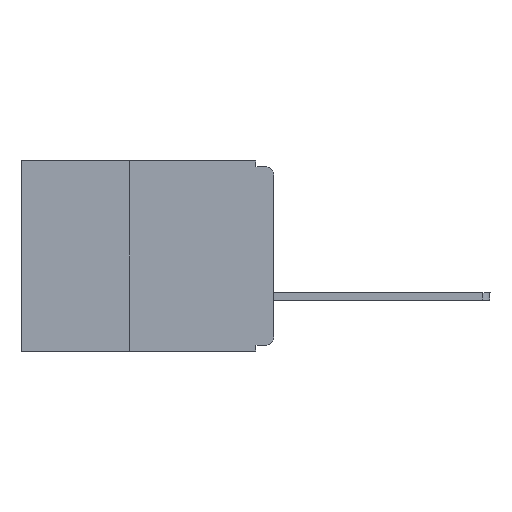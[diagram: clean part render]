
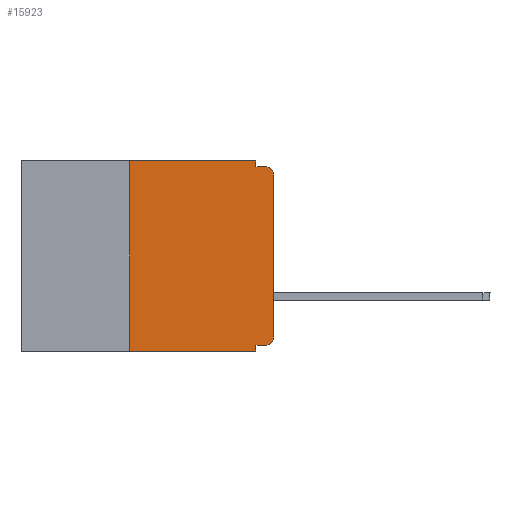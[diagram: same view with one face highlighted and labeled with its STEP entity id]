
A CAD part, left-side view. The second image highlights one B-rep face of the part: STEP entity #15923.
In plain terms, the highlighted planar face has unit normal (-1, 0, 0).
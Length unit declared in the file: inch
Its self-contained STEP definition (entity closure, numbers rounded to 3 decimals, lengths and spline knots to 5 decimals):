
#31 = VECTOR ( 'NONE', #1670, 39.37008 ) ;
#232 = CARTESIAN_POINT ( 'NONE',  ( 0., 0., -0.305 ) ) ;
#716 = CARTESIAN_POINT ( 'NONE',  ( 0., 0.031, -0.01 ) ) ;
#1041 = DIRECTION ( 'NONE',  ( -1., 0., 0. ) ) ;
#1102 = DIRECTION ( 'NONE',  ( 0., 0., -1. ) ) ;
#1212 = ORIENTED_EDGE ( 'NONE', *, *, #5868, .F. ) ;
#1413 = EDGE_CURVE ( 'NONE', #12002, #6217, #3180, .T. ) ;
#1670 = DIRECTION ( 'NONE',  ( 0., 0., 1. ) ) ;
#2000 = LINE ( 'NONE', #8770, #11745 ) ;
#2105 = EDGE_LOOP ( 'NONE', ( #5116, #5267, #5777, #15504, #9404, #3932, #16204, #1212, #5912, #4914 ) ) ;
#2381 = DIRECTION ( 'NONE',  ( 0., 0., -1. ) ) ;
#2387 = DIRECTION ( 'NONE',  ( 1., 0., 0. ) ) ;
#2627 = VERTEX_POINT ( 'NONE', #6374 ) ;
#2690 = CARTESIAN_POINT ( 'NONE',  ( 0., 0.015, -0.305 ) ) ;
#2705 = EDGE_CURVE ( 'NONE', #2627, #14074, #12672, .T. ) ;
#2966 = EDGE_CURVE ( 'NONE', #9240, #2627, #12854, .T. ) ;
#3180 = LINE ( 'NONE', #13560, #15653 ) ;
#3362 = VECTOR ( 'NONE', #7516, 39.37008 ) ;
#3506 = CARTESIAN_POINT ( 'NONE',  ( 0., 0.015, -0.01 ) ) ;
#3932 = ORIENTED_EDGE ( 'NONE', *, *, #13009, .F. ) ;
#4101 = EDGE_CURVE ( 'NONE', #11292, #12118, #8867, .T. ) ;
#4219 = LINE ( 'NONE', #9597, #31 ) ;
#4336 = FACE_OUTER_BOUND ( 'NONE', #2105, .T. ) ;
#4453 = DIRECTION ( 'NONE',  ( 0., 0., 1. ) ) ;
#4914 = ORIENTED_EDGE ( 'NONE', *, *, #14160, .T. ) ;
#5116 = ORIENTED_EDGE ( 'NONE', *, *, #2966, .T. ) ;
#5264 = EDGE_CURVE ( 'NONE', #12173, #6112, #2000, .T. ) ;
#5267 = ORIENTED_EDGE ( 'NONE', *, *, #2705, .T. ) ;
#5777 = ORIENTED_EDGE ( 'NONE', *, *, #9657, .F. ) ;
#5868 = EDGE_CURVE ( 'NONE', #6217, #6112, #9236, .T. ) ;
#5912 = ORIENTED_EDGE ( 'NONE', *, *, #1413, .F. ) ;
#6054 = CARTESIAN_POINT ( 'NONE',  ( 0., 0.031, -0.32 ) ) ;
#6080 = DIRECTION ( 'NONE',  ( 0., -1., 0. ) ) ;
#6112 = VERTEX_POINT ( 'NONE', #16605 ) ;
#6217 = VERTEX_POINT ( 'NONE', #6054 ) ;
#6374 = CARTESIAN_POINT ( 'NONE',  ( 0., 0., -0.025 ) ) ;
#6806 = DIRECTION ( 'NONE',  ( 0., 0., -1. ) ) ;
#7268 = DIRECTION ( 'NONE',  ( 0., -1., 0. ) ) ;
#7516 = DIRECTION ( 'NONE',  ( 0., -1., 0. ) ) ;
#7982 = VERTEX_POINT ( 'NONE', #716 ) ;
#8004 = DIRECTION ( 'NONE',  ( -1., 0., 0. ) ) ;
#8770 = CARTESIAN_POINT ( 'NONE',  ( 0., 0.437, -0.33 ) ) ;
#8867 = LINE ( 'NONE', #14034, #9700 ) ;
#8929 = CARTESIAN_POINT ( 'NONE',  ( 0., 0.015, -0.025 ) ) ;
#9201 = CARTESIAN_POINT ( 'NONE',  ( 0., 0.031, 0. ) ) ;
#9236 = LINE ( 'NONE', #11000, #12559 ) ;
#9240 = VERTEX_POINT ( 'NONE', #232 ) ;
#9404 = ORIENTED_EDGE ( 'NONE', *, *, #4101, .F. ) ;
#9597 = CARTESIAN_POINT ( 'NONE',  ( 0., 0.25, -0.33 ) ) ;
#9657 = EDGE_CURVE ( 'NONE', #7982, #14074, #15204, .T. ) ;
#9700 = VECTOR ( 'NONE', #6080, 39.37008 ) ;
#9705 = CARTESIAN_POINT ( 'NONE',  ( 0., 0.25, 0. ) ) ;
#10078 = CARTESIAN_POINT ( 'NONE',  ( 0., 0.25, -0.33 ) ) ;
#10204 = CARTESIAN_POINT ( 'NONE',  ( 0., 0.015, -0.32 ) ) ;
#11000 = CARTESIAN_POINT ( 'NONE',  ( 0., 0.031, -0.33 ) ) ;
#11209 = VECTOR ( 'NONE', #4453, 39.37008 ) ;
#11210 = VECTOR ( 'NONE', #13467, 39.37008 ) ;
#11292 = VERTEX_POINT ( 'NONE', #9705 ) ;
#11745 = VECTOR ( 'NONE', #7268, 39.37008 ) ;
#11790 = AXIS2_PLACEMENT_3D ( 'NONE', #12886, #2387, #1102 ) ;
#12002 = VERTEX_POINT ( 'NONE', #10204 ) ;
#12029 = CIRCLE ( 'NONE', #14677, 0.015 ) ;
#12118 = VERTEX_POINT ( 'NONE', #9201 ) ;
#12173 = VERTEX_POINT ( 'NONE', #10078 ) ;
#12559 = VECTOR ( 'NONE', #6806, 39.37008 ) ;
#12672 = CIRCLE ( 'NONE', #14644, 0.015 ) ;
#12854 = LINE ( 'NONE', #13676, #11209 ) ;
#12886 = CARTESIAN_POINT ( 'NONE',  ( 0., 0.437, 0. ) ) ;
#13009 = EDGE_CURVE ( 'NONE', #12173, #11292, #4219, .T. ) ;
#13059 = PLANE ( 'NONE',  #11790 ) ;
#13467 = DIRECTION ( 'NONE',  ( 0., 0., -1. ) ) ;
#13560 = CARTESIAN_POINT ( 'NONE',  ( 0., 0., -0.32 ) ) ;
#13620 = DIRECTION ( 'NONE',  ( 0., 1., 0. ) ) ;
#13676 = CARTESIAN_POINT ( 'NONE',  ( 0., 0., 0. ) ) ;
#14034 = CARTESIAN_POINT ( 'NONE',  ( 0., 0.437, 0. ) ) ;
#14074 = VERTEX_POINT ( 'NONE', #3506 ) ;
#14110 = EDGE_CURVE ( 'NONE', #12118, #7982, #14975, .T. ) ;
#14160 = EDGE_CURVE ( 'NONE', #12002, #9240, #12029, .T. ) ;
#14644 = AXIS2_PLACEMENT_3D ( 'NONE', #8929, #1041, #2381 ) ;
#14677 = AXIS2_PLACEMENT_3D ( 'NONE', #2690, #8004, #16036 ) ;
#14975 = LINE ( 'NONE', #16093, #11210 ) ;
#15204 = LINE ( 'NONE', #15561, #3362 ) ;
#15504 = ORIENTED_EDGE ( 'NONE', *, *, #14110, .F. ) ;
#15561 = CARTESIAN_POINT ( 'NONE',  ( 0., 0., -0.01 ) ) ;
#15653 = VECTOR ( 'NONE', #13620, 39.37008 ) ;
#15923 = ADVANCED_FACE ( 'NONE', ( #4336 ), #13059, .F. ) ;
#16036 = DIRECTION ( 'NONE',  ( 0., 0., -1. ) ) ;
#16093 = CARTESIAN_POINT ( 'NONE',  ( 0., 0.031, 0. ) ) ;
#16204 = ORIENTED_EDGE ( 'NONE', *, *, #5264, .T. ) ;
#16605 = CARTESIAN_POINT ( 'NONE',  ( 0., 0.031, -0.33 ) ) ;
